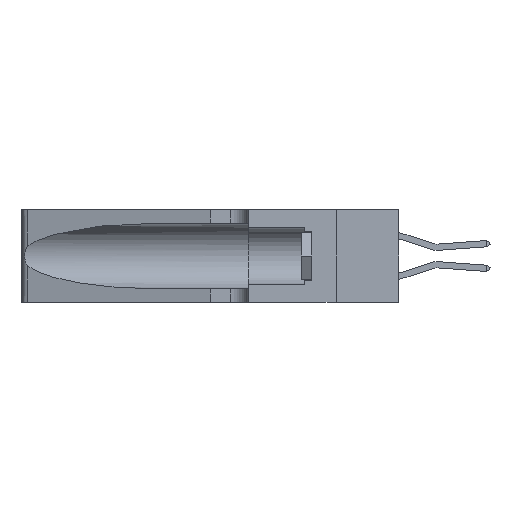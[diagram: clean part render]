
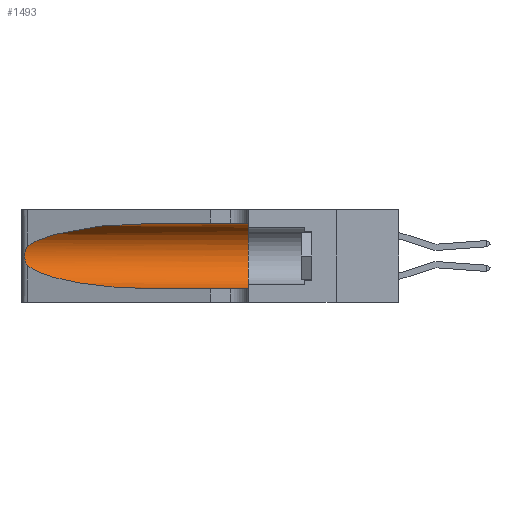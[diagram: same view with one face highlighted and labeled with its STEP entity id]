
A CAD part, left-side view. The second image highlights one B-rep face of the part: STEP entity #1493.
In plain terms, the highlighted cylindrical face has radius 3.308 mm (diameter 6.617 mm), a partial arc.
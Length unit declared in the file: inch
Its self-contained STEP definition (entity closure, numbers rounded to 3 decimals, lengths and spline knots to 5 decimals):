
#155 = ORIENTED_EDGE ( 'NONE', *, *, #9850, .T. ) ;
#1049 = DIRECTION ( 'NONE',  ( 0., 0., -1. ) ) ;
#1296 = DIRECTION ( 'NONE',  ( 0., 1., 0. ) ) ;
#1493 = ADVANCED_FACE ( 'NONE', ( #9472 ), #12394, .F. ) ;
#2450 = EDGE_LOOP ( 'NONE', ( #13675, #155, #16275, #10167, #6191, #21338 ) ) ;
#2573 = CARTESIAN_POINT ( 'NONE',  ( 0.25856, 1.23593, 0.16098 ) ) ;
#2738 = CARTESIAN_POINT ( 'NONE',  ( 0.26017, 1.23833, 0.17102 ) ) ;
#3201 = CARTESIAN_POINT ( 'NONE',  ( 0.1305, 1.61858, 0.31525 ) ) ;
#3328 = CARTESIAN_POINT ( 'NONE',  ( 0.1305, 1.61858, 0.05475 ) ) ;
#3527 = CARTESIAN_POINT ( 'NONE',  ( 0.1305, 0.72297, 0.31525 ) ) ;
#4249 = VECTOR ( 'NONE', #4918, 39.37008 ) ;
#4308 = CARTESIAN_POINT ( 'NONE',  ( 0.25487, 1.22718, 0.22369 ) ) ;
#4390 = CARTESIAN_POINT ( 'NONE',  ( 0.26018, 1.23835, 0.19895 ) ) ;
#4918 = DIRECTION ( 'NONE',  ( 0., -1., 0. ) ) ;
#5115 = CIRCLE ( 'NONE', #21706, 0.13025 ) ;
#6161 = CARTESIAN_POINT ( 'NONE',  ( 0.1305, 1.61858, 0.185 ) ) ;
#6191 = ORIENTED_EDGE ( 'NONE', *, *, #14848, .F. ) ;
#6472 = VECTOR ( 'NONE', #17641, 39.37008 ) ;
#6710 = CARTESIAN_POINT ( 'NONE',  ( 0.1305, 0.35, 0.185 ) ) ;
#8063 = CARTESIAN_POINT ( 'NONE',  ( 0.25854, 1.2359, 0.20912 ) ) ;
#8682 = CARTESIAN_POINT ( 'NONE',  ( 0.25487, 1.22718, 0.22369 ) ) ;
#8993 = CARTESIAN_POINT ( 'NONE',  ( 0.1305, 0.72297, 0.31525 ) ) ;
#9472 = FACE_OUTER_BOUND ( 'NONE', #2450, .T. ) ;
#9508 = CARTESIAN_POINT ( 'NONE',  ( 0.1305, 0.72297, 0.05475 ) ) ;
#9850 = EDGE_CURVE ( 'NONE', #10287, #17172, #15070, .T. ) ;
#10167 = ORIENTED_EDGE ( 'NONE', *, *, #15450, .T. ) ;
#10287 = VERTEX_POINT ( 'NONE', #13080 ) ;
#11453 = CARTESIAN_POINT ( 'NONE',  ( 0.25487, 1.22718, 0.14631 ) ) ;
#11769 = CARTESIAN_POINT ( 'NONE',  ( 0.26075, 1.23896, 0.19203 ) ) ;
#11883 = EDGE_CURVE ( 'NONE', #23308, #10287, #14328, .T. ) ;
#11895 = LINE ( 'NONE', #3201, #4249 ) ;
#11923 = VERTEX_POINT ( 'NONE', #20282 ) ;
#12350 = VERTEX_POINT ( 'NONE', #23525 ) ;
#12394 = CYLINDRICAL_SURFACE ( 'NONE', #19955, 0.13025 ) ;
#12916 = CARTESIAN_POINT ( 'NONE',  ( 0.25487, 1.22718, 0.14631 ) ) ;
#13069 = CARTESIAN_POINT ( 'NONE',  ( 0.18966, 0.96281, 0.05475 ) ) ;
#13080 = CARTESIAN_POINT ( 'NONE',  ( 0.25487, 1.22718, 0.22369 ) ) ;
#13675 = ORIENTED_EDGE ( 'NONE', *, *, #11883, .T. ) ;
#13722 = EDGE_CURVE ( 'NONE', #17172, #11923, #18142, .T. ) ;
#13978 = DIRECTION ( 'NONE',  ( 0., 0., 1. ) ) ;
#14328 =( BOUNDED_CURVE ( )  B_SPLINE_CURVE ( 3, ( #3527, #21402, #19899, #8682 ),
 .UNSPECIFIED., .F., .F. ) 
 B_SPLINE_CURVE_WITH_KNOTS ( ( 4, 4 ),
 ( 1.5708, 2.84003 ),
 .UNSPECIFIED. ) 
 CURVE ( )  GEOMETRIC_REPRESENTATION_ITEM ( )  RATIONAL_B_SPLINE_CURVE ( ( 1., 0.87, 0.87, 1. ) ) 
 REPRESENTATION_ITEM ( '' )  );
#14848 = EDGE_CURVE ( 'NONE', #17812, #12350, #5115, .T. ) ;
#15070 = B_SPLINE_CURVE_WITH_KNOTS ( 'NONE', 3,
 ( #4308, #15292, #19194, #22663, #8063, #4390, #11769, #20925, #2738, #2573, #20849, #18879, #15462, #17285 ),
 .UNSPECIFIED., .F., .F.,
 ( 4, 2, 2, 2, 2, 2, 4 ),
 ( 0., 0.00027, 0.00053, 0.00107, 0.0016, 0.00187, 0.00214 ),
 .UNSPECIFIED. ) ;
#15292 = CARTESIAN_POINT ( 'NONE',  ( 0.25555, 1.22994, 0.2215 ) ) ;
#15450 = EDGE_CURVE ( 'NONE', #11923, #12350, #17341, .T. ) ;
#15462 = CARTESIAN_POINT ( 'NONE',  ( 0.25555, 1.22993, 0.14849 ) ) ;
#16275 = ORIENTED_EDGE ( 'NONE', *, *, #13722, .T. ) ;
#17172 = VERTEX_POINT ( 'NONE', #11453 ) ;
#17285 = CARTESIAN_POINT ( 'NONE',  ( 0.25487, 1.22718, 0.14631 ) ) ;
#17341 = LINE ( 'NONE', #3328, #6472 ) ;
#17641 = DIRECTION ( 'NONE',  ( 0., -1., 0. ) ) ;
#17812 = VERTEX_POINT ( 'NONE', #22406 ) ;
#18142 =( BOUNDED_CURVE ( )  B_SPLINE_CURVE ( 3, ( #12916, #19864, #13069, #9508 ),
 .UNSPECIFIED., .F., .F. ) 
 B_SPLINE_CURVE_WITH_KNOTS ( ( 4, 4 ),
 ( 3.44316, 4.71239 ),
 .UNSPECIFIED. ) 
 CURVE ( )  GEOMETRIC_REPRESENTATION_ITEM ( )  RATIONAL_B_SPLINE_CURVE ( ( 1., 0.87, 0.87, 1. ) ) 
 REPRESENTATION_ITEM ( '' )  );
#18879 = CARTESIAN_POINT ( 'NONE',  ( 0.25639, 1.23186, 0.15144 ) ) ;
#19194 = CARTESIAN_POINT ( 'NONE',  ( 0.25639, 1.23184, 0.21858 ) ) ;
#19864 = CARTESIAN_POINT ( 'NONE',  ( 0.2373, 1.15595, 0.08982 ) ) ;
#19899 = CARTESIAN_POINT ( 'NONE',  ( 0.2373, 1.15595, 0.28018 ) ) ;
#19955 = AXIS2_PLACEMENT_3D ( 'NONE', #6161, #20980, #1049 ) ;
#20282 = CARTESIAN_POINT ( 'NONE',  ( 0.1305, 0.72297, 0.05475 ) ) ;
#20849 = CARTESIAN_POINT ( 'NONE',  ( 0.25789, 1.23486, 0.15765 ) ) ;
#20925 = CARTESIAN_POINT ( 'NONE',  ( 0.26075, 1.23896, 0.178 ) ) ;
#20980 = DIRECTION ( 'NONE',  ( 0., -1., 0. ) ) ;
#21338 = ORIENTED_EDGE ( 'NONE', *, *, #23166, .F. ) ;
#21402 = CARTESIAN_POINT ( 'NONE',  ( 0.18966, 0.96281, 0.31525 ) ) ;
#21706 = AXIS2_PLACEMENT_3D ( 'NONE', #6710, #1296, #13978 ) ;
#22406 = CARTESIAN_POINT ( 'NONE',  ( 0.1305, 0.35, 0.31525 ) ) ;
#22663 = CARTESIAN_POINT ( 'NONE',  ( 0.25787, 1.23484, 0.2124 ) ) ;
#23166 = EDGE_CURVE ( 'NONE', #23308, #17812, #11895, .T. ) ;
#23308 = VERTEX_POINT ( 'NONE', #8993 ) ;
#23525 = CARTESIAN_POINT ( 'NONE',  ( 0.1305, 0.35, 0.05475 ) ) ;
